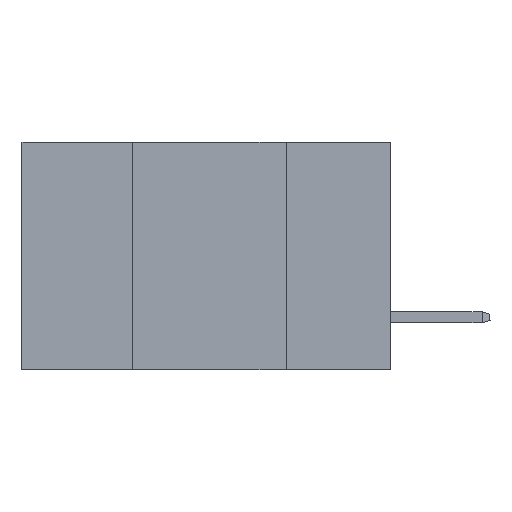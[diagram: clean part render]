
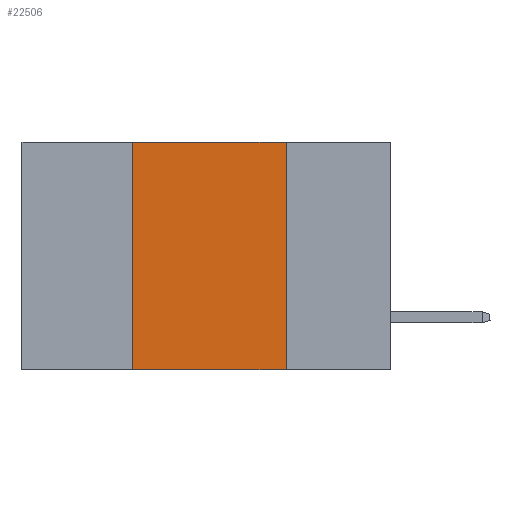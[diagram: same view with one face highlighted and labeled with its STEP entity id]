
A CAD part, left-side view. The second image highlights one B-rep face of the part: STEP entity #22506.
In plain terms, the highlighted planar face has unit normal (-1, 0, 0).
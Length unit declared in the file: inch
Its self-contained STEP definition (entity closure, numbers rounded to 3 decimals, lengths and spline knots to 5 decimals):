
#869 = LINE ( 'NONE', #24328, #17486 ) ;
#1189 = VECTOR ( 'NONE', #2729, 39.37008 ) ;
#2421 = FACE_OUTER_BOUND ( 'NONE', #7344, .T. ) ;
#2729 = DIRECTION ( 'NONE',  ( 0., -1., 0. ) ) ;
#6355 = DIRECTION ( 'NONE',  ( 0., -1., 0. ) ) ;
#7344 = EDGE_LOOP ( 'NONE', ( #21210, #24074, #15803, #8173 ) ) ;
#7862 = EDGE_CURVE ( 'NONE', #22567, #8192, #14277, .T. ) ;
#8173 = ORIENTED_EDGE ( 'NONE', *, *, #7862, .T. ) ;
#8192 = VERTEX_POINT ( 'NONE', #13861 ) ;
#8226 = AXIS2_PLACEMENT_3D ( 'NONE', #15988, #18167, #22030 ) ;
#9503 = CARTESIAN_POINT ( 'NONE',  ( 0., 0.42, -0.37 ) ) ;
#11735 = CARTESIAN_POINT ( 'NONE',  ( 0., 0.6, 0. ) ) ;
#12383 = EDGE_CURVE ( 'NONE', #19479, #8192, #24298, .T. ) ;
#12387 = PLANE ( 'NONE',  #8226 ) ;
#13441 = DIRECTION ( 'NONE',  ( 0., 0., -1. ) ) ;
#13861 = CARTESIAN_POINT ( 'NONE',  ( 0., 0.17, -0.37 ) ) ;
#14118 = CARTESIAN_POINT ( 'NONE',  ( 0., 0.6, -0.37 ) ) ;
#14277 = LINE ( 'NONE', #14118, #22093 ) ;
#14628 = DIRECTION ( 'NONE',  ( 0., 0., 1. ) ) ;
#15803 = ORIENTED_EDGE ( 'NONE', *, *, #17441, .F. ) ;
#15988 = CARTESIAN_POINT ( 'NONE',  ( 0., 0.6, 0. ) ) ;
#17441 = EDGE_CURVE ( 'NONE', #22567, #21730, #869, .T. ) ;
#17486 = VECTOR ( 'NONE', #14628, 39.37008 ) ;
#18167 = DIRECTION ( 'NONE',  ( 1., 0., 0. ) ) ;
#19479 = VERTEX_POINT ( 'NONE', #23090 ) ;
#21210 = ORIENTED_EDGE ( 'NONE', *, *, #12383, .F. ) ;
#21695 = LINE ( 'NONE', #11735, #1189 ) ;
#21730 = VERTEX_POINT ( 'NONE', #23301 ) ;
#22030 = DIRECTION ( 'NONE',  ( 0., 0., -1. ) ) ;
#22093 = VECTOR ( 'NONE', #6355, 39.37008 ) ;
#22506 = ADVANCED_FACE ( 'NONE', ( #2421 ), #12387, .F. ) ;
#22567 = VERTEX_POINT ( 'NONE', #9503 ) ;
#22860 = EDGE_CURVE ( 'NONE', #21730, #19479, #21695, .T. ) ;
#23090 = CARTESIAN_POINT ( 'NONE',  ( 0., 0.17, 0. ) ) ;
#23301 = CARTESIAN_POINT ( 'NONE',  ( 0., 0.42, 0. ) ) ;
#23695 = VECTOR ( 'NONE', #13441, 39.37008 ) ;
#24074 = ORIENTED_EDGE ( 'NONE', *, *, #22860, .F. ) ;
#24298 = LINE ( 'NONE', #24798, #23695 ) ;
#24328 = CARTESIAN_POINT ( 'NONE',  ( 0., 0.42, 0. ) ) ;
#24798 = CARTESIAN_POINT ( 'NONE',  ( 0., 0.17, 0. ) ) ;
